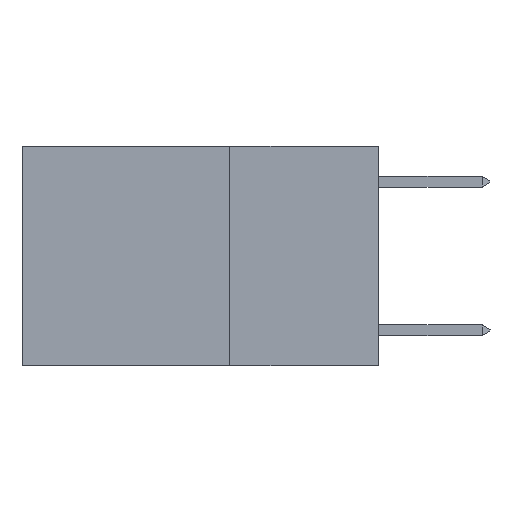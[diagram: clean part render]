
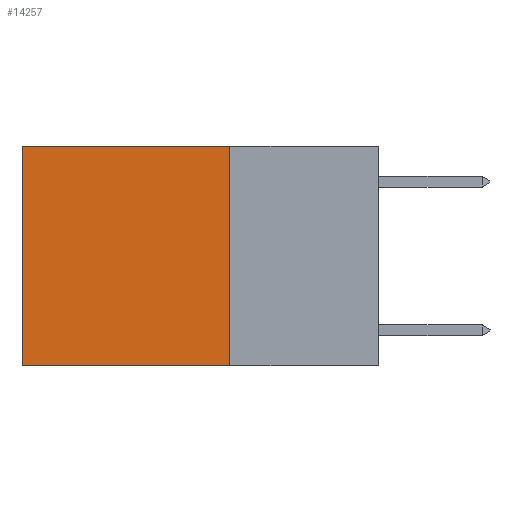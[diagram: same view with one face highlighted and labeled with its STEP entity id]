
A CAD part, left-side view. The second image highlights one B-rep face of the part: STEP entity #14257.
In plain terms, the highlighted planar face has unit normal (-1, 0, 0).
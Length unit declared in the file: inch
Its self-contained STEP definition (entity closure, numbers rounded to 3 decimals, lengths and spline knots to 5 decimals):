
#113 = EDGE_CURVE ( 'NONE', #1407, #6124, #2278, .T. ) ;
#439 = VECTOR ( 'NONE', #15035, 39.37008 ) ;
#659 = PLANE ( 'NONE',  #16635 ) ;
#687 = ORIENTED_EDGE ( 'NONE', *, *, #5127, .F. ) ;
#1407 = VERTEX_POINT ( 'NONE', #14199 ) ;
#1605 = CARTESIAN_POINT ( 'NONE',  ( 0.2625, 0.25, -0.37 ) ) ;
#2278 = LINE ( 'NONE', #3679, #9460 ) ;
#2929 = LINE ( 'NONE', #5855, #439 ) ;
#3679 = CARTESIAN_POINT ( 'NONE',  ( 0.2625, 0.25, 0. ) ) ;
#4342 = CARTESIAN_POINT ( 'NONE',  ( 0.2625, 0.6, -0.37 ) ) ;
#4829 = CARTESIAN_POINT ( 'NONE',  ( 0.2625, 0.6, 0. ) ) ;
#5026 = ORIENTED_EDGE ( 'NONE', *, *, #113, .T. ) ;
#5127 = EDGE_CURVE ( 'NONE', #1407, #5641, #2929, .T. ) ;
#5641 = VERTEX_POINT ( 'NONE', #1605 ) ;
#5855 = CARTESIAN_POINT ( 'NONE',  ( 0.2625, 0.25, 0. ) ) ;
#5870 = DIRECTION ( 'NONE',  ( 1., 0., 0. ) ) ;
#6124 = VERTEX_POINT ( 'NONE', #11386 ) ;
#7860 = LINE ( 'NONE', #4829, #12839 ) ;
#9460 = VECTOR ( 'NONE', #14195, 39.37008 ) ;
#9709 = ORIENTED_EDGE ( 'NONE', *, *, #14526, .T. ) ;
#10033 = ORIENTED_EDGE ( 'NONE', *, *, #19049, .F. ) ;
#11025 = VECTOR ( 'NONE', #18730, 39.37008 ) ;
#11282 = CARTESIAN_POINT ( 'NONE',  ( 0.2625, 0.25, -0.37 ) ) ;
#11386 = CARTESIAN_POINT ( 'NONE',  ( 0.2625, 0.6, 0. ) ) ;
#12086 = DIRECTION ( 'NONE',  ( 0., 0., -1. ) ) ;
#12839 = VECTOR ( 'NONE', #16729, 39.37008 ) ;
#12976 = VERTEX_POINT ( 'NONE', #4342 ) ;
#14195 = DIRECTION ( 'NONE',  ( 0., 1., 0. ) ) ;
#14199 = CARTESIAN_POINT ( 'NONE',  ( 0.2625, 0.25, 0. ) ) ;
#14257 = ADVANCED_FACE ( 'NONE', ( #14360 ), #659, .F. ) ;
#14360 = FACE_OUTER_BOUND ( 'NONE', #19661, .T. ) ;
#14526 = EDGE_CURVE ( 'NONE', #6124, #12976, #7860, .T. ) ;
#15035 = DIRECTION ( 'NONE',  ( 0., 0., -1. ) ) ;
#16542 = CARTESIAN_POINT ( 'NONE',  ( 0.2625, 0.25, 0. ) ) ;
#16635 = AXIS2_PLACEMENT_3D ( 'NONE', #16542, #5870, #12086 ) ;
#16729 = DIRECTION ( 'NONE',  ( 0., 0., -1. ) ) ;
#17234 = LINE ( 'NONE', #11282, #11025 ) ;
#18730 = DIRECTION ( 'NONE',  ( 0., 1., 0. ) ) ;
#19049 = EDGE_CURVE ( 'NONE', #5641, #12976, #17234, .T. ) ;
#19661 = EDGE_LOOP ( 'NONE', ( #9709, #10033, #687, #5026 ) ) ;
